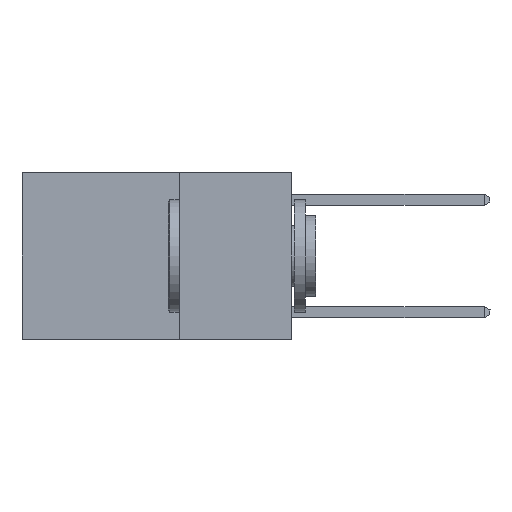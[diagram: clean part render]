
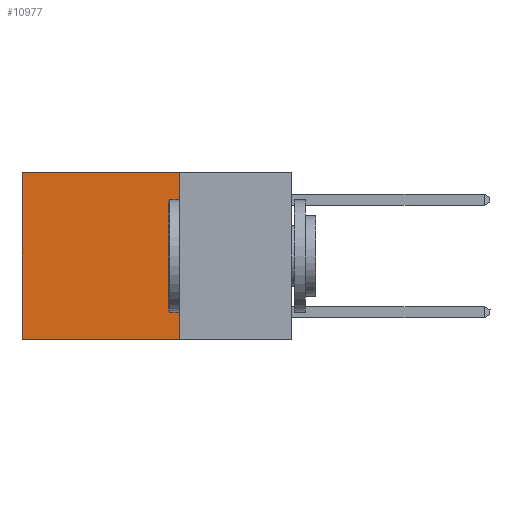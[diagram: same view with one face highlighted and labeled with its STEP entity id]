
A CAD part, left-side view. The second image highlights one B-rep face of the part: STEP entity #10977.
In plain terms, the highlighted planar face has unit normal (-1, 0, 0).
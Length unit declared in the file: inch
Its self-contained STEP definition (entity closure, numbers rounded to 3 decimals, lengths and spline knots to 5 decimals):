
#63 = CARTESIAN_POINT ( 'NONE',  ( 0.2625, 0.25, 0. ) ) ;
#112 = LINE ( 'NONE', #5212, #13247 ) ;
#175 = ORIENTED_EDGE ( 'NONE', *, *, #9687, .T. ) ;
#1873 = VECTOR ( 'NONE', #11067, 39.37008 ) ;
#2049 = EDGE_CURVE ( 'NONE', #3615, #7255, #6673, .T. ) ;
#2060 = DIRECTION ( 'NONE',  ( 1., 0., 0. ) ) ;
#2097 = EDGE_CURVE ( 'NONE', #13905, #7255, #112, .T. ) ;
#2438 = DIRECTION ( 'NONE',  ( 0., 1., 0. ) ) ;
#3233 = CARTESIAN_POINT ( 'NONE',  ( 0.2625, 0.25, 0. ) ) ;
#3615 = VERTEX_POINT ( 'NONE', #5768 ) ;
#4213 = VECTOR ( 'NONE', #2438, 39.37008 ) ;
#4390 = CARTESIAN_POINT ( 'NONE',  ( 0.2625, 0.25, 0. ) ) ;
#4688 = ORIENTED_EDGE ( 'NONE', *, *, #2049, .F. ) ;
#5212 = CARTESIAN_POINT ( 'NONE',  ( 0.2625, 0.6, 0. ) ) ;
#5768 = CARTESIAN_POINT ( 'NONE',  ( 0.2625, 0.25, -0.37 ) ) ;
#6673 = LINE ( 'NONE', #8505, #12544 ) ;
#6982 = EDGE_CURVE ( 'NONE', #12419, #3615, #11271, .T. ) ;
#7176 = LINE ( 'NONE', #12451, #4213 ) ;
#7188 = AXIS2_PLACEMENT_3D ( 'NONE', #4390, #2060, #10004 ) ;
#7255 = VERTEX_POINT ( 'NONE', #10286 ) ;
#7453 = DIRECTION ( 'NONE',  ( 0., 0., -1. ) ) ;
#7756 = PLANE ( 'NONE',  #7188 ) ;
#8016 = EDGE_LOOP ( 'NONE', ( #12854, #4688, #13741, #175 ) ) ;
#8505 = CARTESIAN_POINT ( 'NONE',  ( 0.2625, 0.25, -0.37 ) ) ;
#9609 = DIRECTION ( 'NONE',  ( 0., 1., 0. ) ) ;
#9687 = EDGE_CURVE ( 'NONE', #12419, #13905, #7176, .T. ) ;
#10004 = DIRECTION ( 'NONE',  ( 0., 0., -1. ) ) ;
#10286 = CARTESIAN_POINT ( 'NONE',  ( 0.2625, 0.6, -0.37 ) ) ;
#10977 = ADVANCED_FACE ( 'NONE', ( #12345 ), #7756, .F. ) ;
#11067 = DIRECTION ( 'NONE',  ( 0., 0., -1. ) ) ;
#11271 = LINE ( 'NONE', #3233, #1873 ) ;
#12252 = CARTESIAN_POINT ( 'NONE',  ( 0.2625, 0.6, 0. ) ) ;
#12345 = FACE_OUTER_BOUND ( 'NONE', #8016, .T. ) ;
#12419 = VERTEX_POINT ( 'NONE', #63 ) ;
#12451 = CARTESIAN_POINT ( 'NONE',  ( 0.2625, 0.25, 0. ) ) ;
#12544 = VECTOR ( 'NONE', #9609, 39.37008 ) ;
#12854 = ORIENTED_EDGE ( 'NONE', *, *, #2097, .T. ) ;
#13247 = VECTOR ( 'NONE', #7453, 39.37008 ) ;
#13741 = ORIENTED_EDGE ( 'NONE', *, *, #6982, .F. ) ;
#13905 = VERTEX_POINT ( 'NONE', #12252 ) ;
